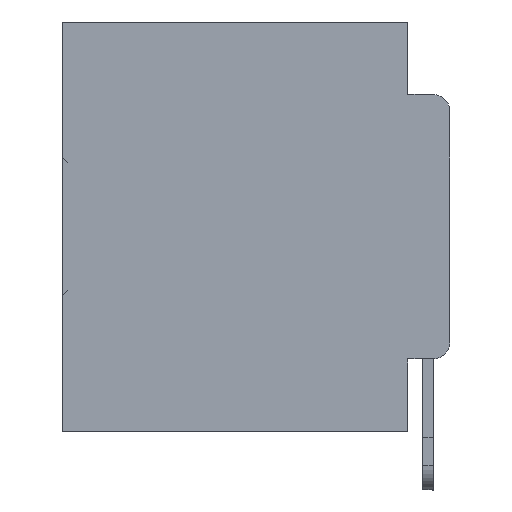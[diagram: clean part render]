
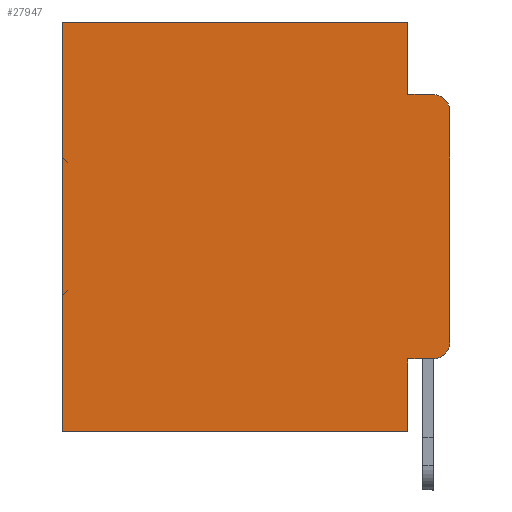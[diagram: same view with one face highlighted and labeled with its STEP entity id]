
A CAD part, left-side view. The second image highlights one B-rep face of the part: STEP entity #27947.
In plain terms, the highlighted planar face has unit normal (-1, 0, 0).
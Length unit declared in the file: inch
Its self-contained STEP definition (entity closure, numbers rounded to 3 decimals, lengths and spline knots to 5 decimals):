
#175 = VECTOR ( 'NONE', #26096, 39.37008 ) ;
#240 = CARTESIAN_POINT ( 'NONE',  ( 0.298, 0.051, -0.0885 ) ) ;
#2097 = EDGE_LOOP ( 'NONE', ( #20712, #10731, #16223, #6942, #2736, #20891, #23981, #2834, #25319, #21409 ) ) ;
#2370 = DIRECTION ( 'NONE',  ( 0., 0., -1. ) ) ;
#2736 = ORIENTED_EDGE ( 'NONE', *, *, #3007, .T. ) ;
#2765 = AXIS2_PLACEMENT_3D ( 'NONE', #30035, #8208, #19296 ) ;
#2834 = ORIENTED_EDGE ( 'NONE', *, *, #6858, .F. ) ;
#3007 = EDGE_CURVE ( 'NONE', #4899, #24377, #20168, .T. ) ;
#3329 = LINE ( 'NONE', #16968, #35863 ) ;
#4119 = VERTEX_POINT ( 'NONE', #26380 ) ;
#4899 = VERTEX_POINT ( 'NONE', #25745 ) ;
#5031 = PLANE ( 'NONE',  #28872 ) ;
#5221 = VERTEX_POINT ( 'NONE', #240 ) ;
#5366 = CARTESIAN_POINT ( 'NONE',  ( 0.298, 0., -0.1085 ) ) ;
#6213 = CARTESIAN_POINT ( 'NONE',  ( 0.298, 0., 0. ) ) ;
#6518 = CARTESIAN_POINT ( 'NONE',  ( 0.298, 0., 0. ) ) ;
#6858 = EDGE_CURVE ( 'NONE', #9675, #4119, #18569, .T. ) ;
#6942 = ORIENTED_EDGE ( 'NONE', *, *, #13644, .F. ) ;
#6951 = CARTESIAN_POINT ( 'NONE',  ( 0.298, 0.051, -0.0885 ) ) ;
#8204 = VECTOR ( 'NONE', #2370, 39.37008 ) ;
#8208 = DIRECTION ( 'NONE',  ( -1., 0., 0. ) ) ;
#9675 = VERTEX_POINT ( 'NONE', #16698 ) ;
#10731 = ORIENTED_EDGE ( 'NONE', *, *, #31496, .T. ) ;
#12043 = DIRECTION ( 'NONE',  ( 0., 0., -1. ) ) ;
#12221 = DIRECTION ( 'NONE',  ( -1., 0., 0. ) ) ;
#12735 = EDGE_CURVE ( 'NONE', #5221, #25800, #14956, .T. ) ;
#13644 = EDGE_CURVE ( 'NONE', #4899, #5221, #23995, .T. ) ;
#13707 = VECTOR ( 'NONE', #15239, 39.37008 ) ;
#13854 = DIRECTION ( 'NONE',  ( 0., 0., -1. ) ) ;
#14085 = CARTESIAN_POINT ( 'NONE',  ( 0.298, 0., 0. ) ) ;
#14956 = LINE ( 'NONE', #6951, #35629 ) ;
#15239 = DIRECTION ( 'NONE',  ( 0., 1., 0. ) ) ;
#15663 = CARTESIAN_POINT ( 'NONE',  ( 0.298, 0.051, 0. ) ) ;
#15690 = CARTESIAN_POINT ( 'NONE',  ( 0.298, 0.473, 0. ) ) ;
#16223 = ORIENTED_EDGE ( 'NONE', *, *, #12735, .F. ) ;
#16316 = FACE_OUTER_BOUND ( 'NONE', #2097, .T. ) ;
#16698 = CARTESIAN_POINT ( 'NONE',  ( 0.298, 0.051, -0.4115 ) ) ;
#16968 = CARTESIAN_POINT ( 'NONE',  ( 0.298, 0., -0.5 ) ) ;
#17008 = VECTOR ( 'NONE', #32189, 39.37008 ) ;
#17141 = VERTEX_POINT ( 'NONE', #34902 ) ;
#17562 = EDGE_CURVE ( 'NONE', #9675, #17141, #27054, .T. ) ;
#18194 = EDGE_CURVE ( 'NONE', #35449, #19250, #20208, .T. ) ;
#18569 = LINE ( 'NONE', #15663, #8204 ) ;
#19250 = VERTEX_POINT ( 'NONE', #21378 ) ;
#19296 = DIRECTION ( 'NONE',  ( 0., 0., -1. ) ) ;
#20168 = LINE ( 'NONE', #6518, #13707 ) ;
#20208 = LINE ( 'NONE', #6213, #34850 ) ;
#20417 = VERTEX_POINT ( 'NONE', #28972 ) ;
#20712 = ORIENTED_EDGE ( 'NONE', *, *, #18194, .F. ) ;
#20891 = ORIENTED_EDGE ( 'NONE', *, *, #29350, .T. ) ;
#21089 = CARTESIAN_POINT ( 'NONE',  ( 0.298, 0.051, 0. ) ) ;
#21231 = DIRECTION ( 'NONE',  ( 0., -1., 0. ) ) ;
#21378 = CARTESIAN_POINT ( 'NONE',  ( 0.298, 0., -0.3915 ) ) ;
#21409 = ORIENTED_EDGE ( 'NONE', *, *, #34843, .T. ) ;
#23981 = ORIENTED_EDGE ( 'NONE', *, *, #34568, .F. ) ;
#23995 = LINE ( 'NONE', #21089, #17008 ) ;
#24062 = CIRCLE ( 'NONE', #27529, 0.02 ) ;
#24377 = VERTEX_POINT ( 'NONE', #15690 ) ;
#25303 = CARTESIAN_POINT ( 'NONE',  ( 0.298, 0.02, -0.1085 ) ) ;
#25319 = ORIENTED_EDGE ( 'NONE', *, *, #17562, .T. ) ;
#25745 = CARTESIAN_POINT ( 'NONE',  ( 0.298, 0.051, 0. ) ) ;
#25800 = VERTEX_POINT ( 'NONE', #33130 ) ;
#26096 = DIRECTION ( 'NONE',  ( 0., 0., -1. ) ) ;
#26380 = CARTESIAN_POINT ( 'NONE',  ( 0.298, 0.051, -0.5 ) ) ;
#27054 = LINE ( 'NONE', #32501, #34824 ) ;
#27529 = AXIS2_PLACEMENT_3D ( 'NONE', #25303, #12221, #12043 ) ;
#27907 = DIRECTION ( 'NONE',  ( 1., 0., 0. ) ) ;
#27947 = ADVANCED_FACE ( 'NONE', ( #16316 ), #5031, .F. ) ;
#28872 = AXIS2_PLACEMENT_3D ( 'NONE', #14085, #27907, #30470 ) ;
#28972 = CARTESIAN_POINT ( 'NONE',  ( 0.298, 0.473, -0.5 ) ) ;
#29350 = EDGE_CURVE ( 'NONE', #24377, #20417, #34269, .T. ) ;
#30035 = CARTESIAN_POINT ( 'NONE',  ( 0.298, 0.02, -0.3915 ) ) ;
#30470 = DIRECTION ( 'NONE',  ( 0., 0., -1. ) ) ;
#31189 = CARTESIAN_POINT ( 'NONE',  ( 0.298, 0.473, 0. ) ) ;
#31315 = DIRECTION ( 'NONE',  ( 0., -1., 0. ) ) ;
#31496 = EDGE_CURVE ( 'NONE', #35449, #25800, #24062, .T. ) ;
#32189 = DIRECTION ( 'NONE',  ( 0., 0., -1. ) ) ;
#32501 = CARTESIAN_POINT ( 'NONE',  ( 0.298, 0.051, -0.4115 ) ) ;
#33130 = CARTESIAN_POINT ( 'NONE',  ( 0.298, 0.02, -0.0885 ) ) ;
#33329 = DIRECTION ( 'NONE',  ( 0., 1., 0. ) ) ;
#34111 = CIRCLE ( 'NONE', #2765, 0.02 ) ;
#34269 = LINE ( 'NONE', #31189, #175 ) ;
#34568 = EDGE_CURVE ( 'NONE', #4119, #20417, #3329, .T. ) ;
#34824 = VECTOR ( 'NONE', #21231, 39.37008 ) ;
#34843 = EDGE_CURVE ( 'NONE', #17141, #19250, #34111, .T. ) ;
#34850 = VECTOR ( 'NONE', #13854, 39.37008 ) ;
#34902 = CARTESIAN_POINT ( 'NONE',  ( 0.298, 0.02, -0.4115 ) ) ;
#35449 = VERTEX_POINT ( 'NONE', #5366 ) ;
#35629 = VECTOR ( 'NONE', #31315, 39.37008 ) ;
#35863 = VECTOR ( 'NONE', #33329, 39.37008 ) ;
